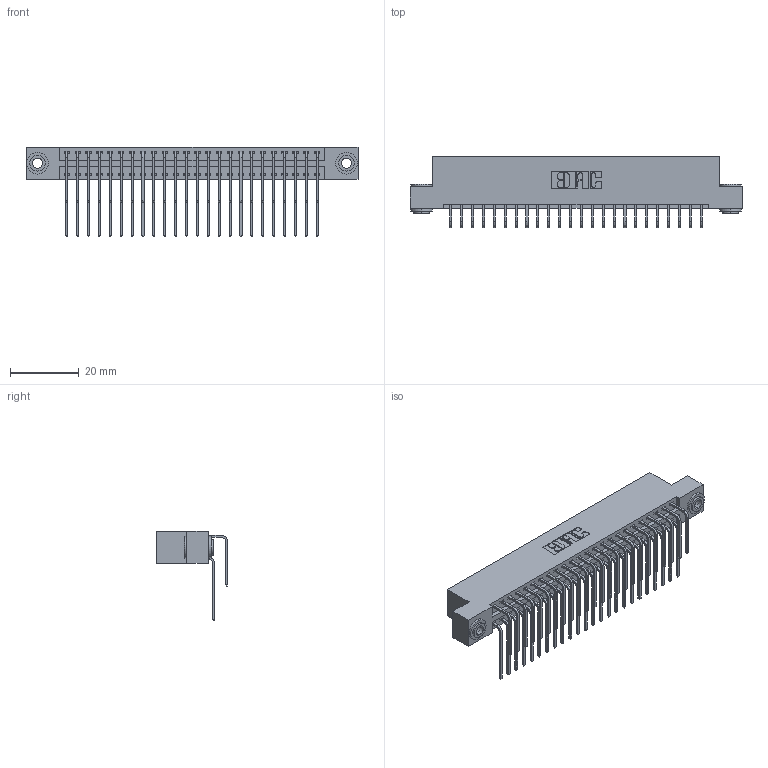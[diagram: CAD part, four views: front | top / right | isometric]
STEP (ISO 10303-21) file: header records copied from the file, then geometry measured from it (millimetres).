
FILE_DESCRIPTION (( 'STEP AP203' ), '1' );
FILE_NAME ('346-048-559-203.STEP', '2022-05-20T22:13:30', ( '' ), ( '' ), 'SwSTEP 2.0', 'SolidWorks 2020', '' );
FILE_SCHEMA (( 'CONFIG_CONTROL_DESIGN' ));
Length unit declared in the file: inch
Products named in the file (5): 346-048-559-203; 345-292-001_559 Tail - 2; 346 Part_Flush Mounting Lugs - 0.156 Dia-TH; 345-250-002_345-250-002-102; 345-292-001_558 559 Tail - 1
Assembly tree (51 placements, depth 2):
  346-048-559-203
    346 Part_Flush Mounting Lugs - 0.156 Dia-TH
    345-292-001_558 559 Tail - 1  x24
    345-292-001_559 Tail - 2  x24
    345-250-002_345-250-002-102  x2
Bounding box: 96.77 x 20.89 x 26.16 mm (x, y, z)
Volume: 9575.1 mm3; surface area: 14455.8 mm2
Topology: 51 solids, 51 shells, 2766 faces, 8169 edges, 5378 vertices
Faces by surface type: plane 1876, cylinder 882, cone 8
Entity records: 20936 total; most frequent: CARTESIAN_POINT 3508, ORIENTED_EDGE 3382, DIRECTION 3145, EDGE_CURVE 1691, VECTOR 1399, LINE 1399, VERTEX_POINT 1122, AXIS2_PLACEMENT_3D 873
